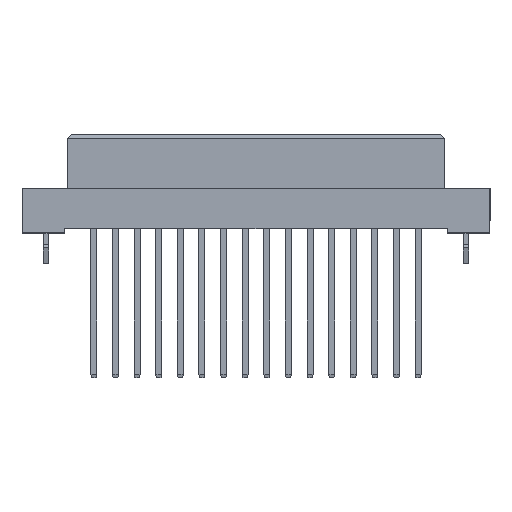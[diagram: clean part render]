
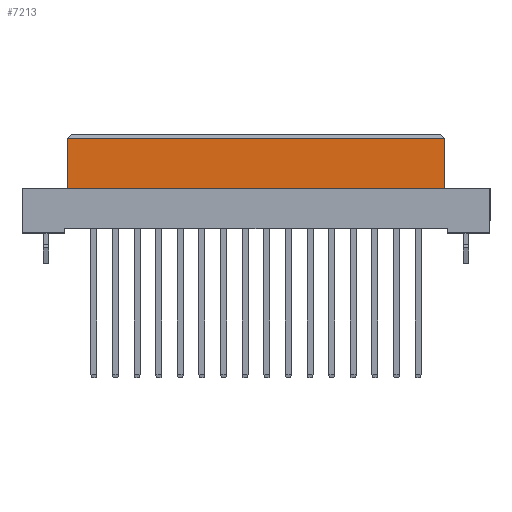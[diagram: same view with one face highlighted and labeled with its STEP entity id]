
A CAD part, top view. The second image highlights one B-rep face of the part: STEP entity #7213.
In plain terms, the highlighted planar face has unit normal (0, 0, 1).
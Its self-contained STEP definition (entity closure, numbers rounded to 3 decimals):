
#67 = CARTESIAN_POINT ( 'NONE',  ( -22.2, -0.5, 4.25 ) ) ;
#1017 = VECTOR ( 'NONE', #11894, 1000. ) ;
#1698 = CARTESIAN_POINT ( 'NONE',  ( -22.2, -6.4, 4.25 ) ) ;
#2215 = CARTESIAN_POINT ( 'NONE',  ( 22.2, -0.5, 4.25 ) ) ;
#2592 = ORIENTED_EDGE ( 'NONE', *, *, #7759, .T. ) ;
#2865 = VERTEX_POINT ( 'NONE', #2215 ) ;
#3024 = DIRECTION ( 'NONE',  ( 0., 0., 1. ) ) ;
#3483 = VECTOR ( 'NONE', #20067, 1000. ) ;
#4643 = CARTESIAN_POINT ( 'NONE',  ( 22.2, -6.4, 4.25 ) ) ;
#6085 = VECTOR ( 'NONE', #17212, 1000. ) ;
#6168 = ORIENTED_EDGE ( 'NONE', *, *, #21148, .F. ) ;
#6681 = LINE ( 'NONE', #13304, #1017 ) ;
#7088 = CARTESIAN_POINT ( 'NONE',  ( 22.2, -6.4, 4.25 ) ) ;
#7213 = ADVANCED_FACE ( 'NONE', ( #16500 ), #16609, .T. ) ;
#7759 = EDGE_CURVE ( 'NONE', #19630, #19656, #6681, .T. ) ;
#11412 = AXIS2_PLACEMENT_3D ( 'NONE', #4643, #3024, #18130 ) ;
#11588 = LINE ( 'NONE', #1698, #19845 ) ;
#11699 = EDGE_LOOP ( 'NONE', ( #17380, #17538, #6168, #2592 ) ) ;
#11894 = DIRECTION ( 'NONE',  ( 1., 0., 0. ) ) ;
#12077 = LINE ( 'NONE', #7088, #6085 ) ;
#12466 = VERTEX_POINT ( 'NONE', #15779 ) ;
#13304 = CARTESIAN_POINT ( 'NONE',  ( 22.2, -6.4, 4.25 ) ) ;
#14969 = LINE ( 'NONE', #67, #3483 ) ;
#15412 = CARTESIAN_POINT ( 'NONE',  ( -22.2, -6.4, 4.25 ) ) ;
#15636 = CARTESIAN_POINT ( 'NONE',  ( 22.2, -6.4, 4.25 ) ) ;
#15779 = CARTESIAN_POINT ( 'NONE',  ( -22.2, -0.5, 4.25 ) ) ;
#16403 = EDGE_CURVE ( 'NONE', #2865, #12466, #14969, .T. ) ;
#16500 = FACE_OUTER_BOUND ( 'NONE', #11699, .T. ) ;
#16609 = PLANE ( 'NONE',  #11412 ) ;
#17212 = DIRECTION ( 'NONE',  ( 0., 1., 0. ) ) ;
#17380 = ORIENTED_EDGE ( 'NONE', *, *, #18571, .T. ) ;
#17538 = ORIENTED_EDGE ( 'NONE', *, *, #16403, .T. ) ;
#18130 = DIRECTION ( 'NONE',  ( 1., 0., 0. ) ) ;
#18571 = EDGE_CURVE ( 'NONE', #19656, #2865, #12077, .T. ) ;
#19630 = VERTEX_POINT ( 'NONE', #15412 ) ;
#19656 = VERTEX_POINT ( 'NONE', #15636 ) ;
#19845 = VECTOR ( 'NONE', #20069, 1000. ) ;
#20067 = DIRECTION ( 'NONE',  ( -1., 0., 0. ) ) ;
#20069 = DIRECTION ( 'NONE',  ( 0., 1., 0. ) ) ;
#21148 = EDGE_CURVE ( 'NONE', #19630, #12466, #11588, .T. ) ;
